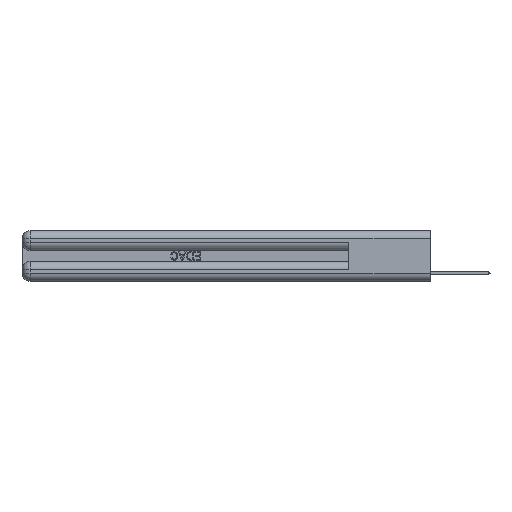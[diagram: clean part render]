
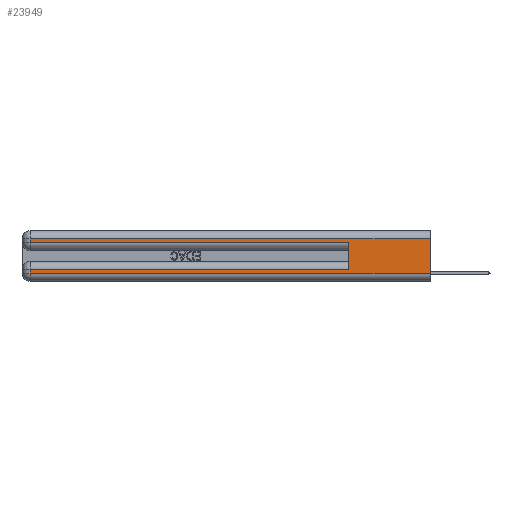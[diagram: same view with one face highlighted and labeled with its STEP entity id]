
A CAD part, left-side view. The second image highlights one B-rep face of the part: STEP entity #23949.
In plain terms, the highlighted planar face has unit normal (-1, 0, 0).
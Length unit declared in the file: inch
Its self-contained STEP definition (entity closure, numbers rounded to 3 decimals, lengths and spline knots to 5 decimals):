
#798 = DIRECTION ( 'NONE',  ( 0., 0., -1. ) ) ;
#817 = CARTESIAN_POINT ( 'NONE',  ( 0., 0., 0.31 ) ) ;
#1010 = DIRECTION ( 'NONE',  ( 0., 1., 0. ) ) ;
#1186 = CARTESIAN_POINT ( 'NONE',  ( 0., 0., 0.285 ) ) ;
#1294 = EDGE_CURVE ( 'NONE', #11731, #13541, #20273, .T. ) ;
#1446 = EDGE_CURVE ( 'NONE', #8023, #11731, #14584, .T. ) ;
#1557 = VECTOR ( 'NONE', #14773, 39.37008 ) ;
#3405 = LINE ( 'NONE', #26498, #18729 ) ;
#3482 = ORIENTED_EDGE ( 'NONE', *, *, #9354, .T. ) ;
#3660 = EDGE_CURVE ( 'NONE', #9613, #8023, #22897, .T. ) ;
#4000 = CARTESIAN_POINT ( 'NONE',  ( 0., 0.6, 0.145 ) ) ;
#4325 = ORIENTED_EDGE ( 'NONE', *, *, #1446, .T. ) ;
#4949 = ORIENTED_EDGE ( 'NONE', *, *, #1294, .T. ) ;
#5014 = CARTESIAN_POINT ( 'NONE',  ( 0., 0., 0.085 ) ) ;
#5709 = ORIENTED_EDGE ( 'NONE', *, *, #24395, .T. ) ;
#5937 = LINE ( 'NONE', #4000, #15223 ) ;
#6104 = CARTESIAN_POINT ( 'NONE',  ( 0., 0., 0.06 ) ) ;
#6219 = DIRECTION ( 'NONE',  ( 0., 0., 1. ) ) ;
#6353 = CARTESIAN_POINT ( 'NONE',  ( 0., 0., 0.06 ) ) ;
#7234 = CARTESIAN_POINT ( 'NONE',  ( 0., 2.94, 0.31 ) ) ;
#7669 = DIRECTION ( 'NONE',  ( 0., -1., 0. ) ) ;
#7790 = VECTOR ( 'NONE', #8224, 39.37008 ) ;
#8023 = VERTEX_POINT ( 'NONE', #7234 ) ;
#8224 = DIRECTION ( 'NONE',  ( 0., 0., -1. ) ) ;
#8913 = CARTESIAN_POINT ( 'NONE',  ( 0., 2.94, 0.085 ) ) ;
#9354 = EDGE_CURVE ( 'NONE', #17044, #25174, #15658, .T. ) ;
#9613 = VERTEX_POINT ( 'NONE', #817 ) ;
#10002 = CARTESIAN_POINT ( 'NONE',  ( 0., 0.6, 0.085 ) ) ;
#10125 = CARTESIAN_POINT ( 'NONE',  ( 0., 2.94, 0.06 ) ) ;
#10264 = DIRECTION ( 'NONE',  ( 0., 0., -1. ) ) ;
#10512 = ORIENTED_EDGE ( 'NONE', *, *, #24428, .F. ) ;
#11321 = ORIENTED_EDGE ( 'NONE', *, *, #3660, .T. ) ;
#11731 = VERTEX_POINT ( 'NONE', #14171 ) ;
#11881 = DIRECTION ( 'NONE',  ( 0., 1., 0. ) ) ;
#12154 = AXIS2_PLACEMENT_3D ( 'NONE', #18836, #23384, #10264 ) ;
#12549 = DIRECTION ( 'NONE',  ( 0., 0., -1. ) ) ;
#12680 = EDGE_CURVE ( 'NONE', #25174, #25270, #20573, .T. ) ;
#12768 = EDGE_CURVE ( 'NONE', #9613, #13263, #3405, .T. ) ;
#12980 = VECTOR ( 'NONE', #12549, 39.37008 ) ;
#13263 = VERTEX_POINT ( 'NONE', #6104 ) ;
#13399 = CARTESIAN_POINT ( 'NONE',  ( 0., 0.6, 0.285 ) ) ;
#13541 = VERTEX_POINT ( 'NONE', #13399 ) ;
#14171 = CARTESIAN_POINT ( 'NONE',  ( 0., 2.94, 0.285 ) ) ;
#14584 = LINE ( 'NONE', #24951, #7790 ) ;
#14621 = VECTOR ( 'NONE', #1010, 39.37008 ) ;
#14773 = DIRECTION ( 'NONE',  ( 0., -1., 0. ) ) ;
#15223 = VECTOR ( 'NONE', #6219, 39.37008 ) ;
#15658 = LINE ( 'NONE', #5014, #14621 ) ;
#15747 = VECTOR ( 'NONE', #7669, 39.37008 ) ;
#17044 = VERTEX_POINT ( 'NONE', #10002 ) ;
#17664 = EDGE_LOOP ( 'NONE', ( #17761, #11321, #4325, #4949, #10512, #3482, #26448, #5709 ) ) ;
#17761 = ORIENTED_EDGE ( 'NONE', *, *, #12768, .F. ) ;
#18729 = VECTOR ( 'NONE', #798, 39.37008 ) ;
#18836 = CARTESIAN_POINT ( 'NONE',  ( 0., 0., 0.37 ) ) ;
#20273 = LINE ( 'NONE', #1186, #15747 ) ;
#20573 = LINE ( 'NONE', #22511, #12980 ) ;
#21983 = CARTESIAN_POINT ( 'NONE',  ( 0., 0., 0.31 ) ) ;
#22511 = CARTESIAN_POINT ( 'NONE',  ( 0., 2.94, 0.37 ) ) ;
#22897 = LINE ( 'NONE', #21983, #23006 ) ;
#22984 = FACE_OUTER_BOUND ( 'NONE', #17664, .T. ) ;
#23006 = VECTOR ( 'NONE', #11881, 39.37008 ) ;
#23245 = PLANE ( 'NONE',  #12154 ) ;
#23384 = DIRECTION ( 'NONE',  ( 1., 0., 0. ) ) ;
#23949 = ADVANCED_FACE ( 'NONE', ( #22984 ), #23245, .F. ) ;
#24395 = EDGE_CURVE ( 'NONE', #25270, #13263, #25418, .T. ) ;
#24428 = EDGE_CURVE ( 'NONE', #17044, #13541, #5937, .T. ) ;
#24951 = CARTESIAN_POINT ( 'NONE',  ( 0., 2.94, 0.37 ) ) ;
#25174 = VERTEX_POINT ( 'NONE', #8913 ) ;
#25270 = VERTEX_POINT ( 'NONE', #10125 ) ;
#25418 = LINE ( 'NONE', #6353, #1557 ) ;
#26448 = ORIENTED_EDGE ( 'NONE', *, *, #12680, .T. ) ;
#26498 = CARTESIAN_POINT ( 'NONE',  ( 0., 0., 0.37 ) ) ;
